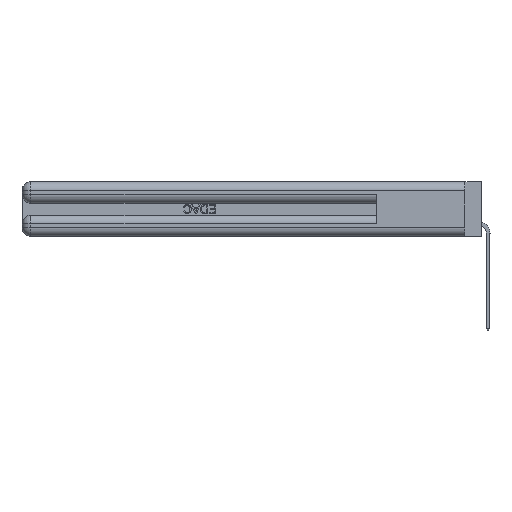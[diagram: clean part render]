
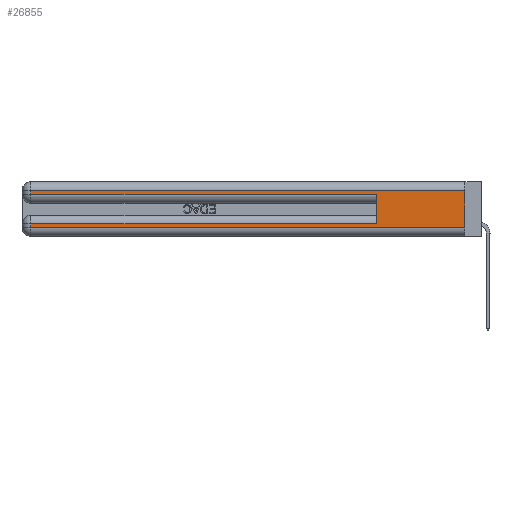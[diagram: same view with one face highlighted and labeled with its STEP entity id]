
A CAD part, left-side view. The second image highlights one B-rep face of the part: STEP entity #26855.
In plain terms, the highlighted planar face has unit normal (-1, 0, 0).
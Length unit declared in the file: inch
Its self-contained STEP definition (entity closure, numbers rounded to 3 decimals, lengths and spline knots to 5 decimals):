
#273 = CARTESIAN_POINT ( 'NONE',  ( 0., 0.6, 0.145 ) ) ;
#765 = ORIENTED_EDGE ( 'NONE', *, *, #25468, .F. ) ;
#1074 = VERTEX_POINT ( 'NONE', #37345 ) ;
#1900 = VECTOR ( 'NONE', #47038, 39.37008 ) ;
#2160 = VECTOR ( 'NONE', #4146, 39.37008 ) ;
#3817 = VECTOR ( 'NONE', #32555, 39.37008 ) ;
#4146 = DIRECTION ( 'NONE',  ( 0., 0., 1. ) ) ;
#4957 = ORIENTED_EDGE ( 'NONE', *, *, #15949, .F. ) ;
#7104 = CARTESIAN_POINT ( 'NONE',  ( 0., 2.94, 0.37 ) ) ;
#8196 = PLANE ( 'NONE',  #9408 ) ;
#8987 = LINE ( 'NONE', #21500, #15284 ) ;
#9408 = AXIS2_PLACEMENT_3D ( 'NONE', #19768, #37480, #22965 ) ;
#9443 = EDGE_LOOP ( 'NONE', ( #765, #43252, #29147, #25705, #4957, #15917, #16515, #45748 ) ) ;
#9847 = VERTEX_POINT ( 'NONE', #37475 ) ;
#10037 = VERTEX_POINT ( 'NONE', #35838 ) ;
#12212 = EDGE_CURVE ( 'NONE', #10037, #40613, #35319, .T. ) ;
#14275 = LINE ( 'NONE', #273, #2160 ) ;
#14607 = LINE ( 'NONE', #45382, #1900 ) ;
#14815 = CARTESIAN_POINT ( 'NONE',  ( 0., 0., 0.285 ) ) ;
#15149 = LINE ( 'NONE', #35776, #22047 ) ;
#15284 = VECTOR ( 'NONE', #17341, 39.37008 ) ;
#15917 = ORIENTED_EDGE ( 'NONE', *, *, #21613, .T. ) ;
#15949 = EDGE_CURVE ( 'NONE', #1074, #41751, #14275, .T. ) ;
#16515 = ORIENTED_EDGE ( 'NONE', *, *, #39843, .T. ) ;
#16596 = VERTEX_POINT ( 'NONE', #25497 ) ;
#17341 = DIRECTION ( 'NONE',  ( 0., 1., 0. ) ) ;
#18153 = VECTOR ( 'NONE', #25629, 39.37008 ) ;
#19569 = VERTEX_POINT ( 'NONE', #19825 ) ;
#19768 = CARTESIAN_POINT ( 'NONE',  ( 0., 0., 0.37 ) ) ;
#19825 = CARTESIAN_POINT ( 'NONE',  ( 0., 2.94, 0.285 ) ) ;
#21500 = CARTESIAN_POINT ( 'NONE',  ( 0., 0., 0.31 ) ) ;
#21613 = EDGE_CURVE ( 'NONE', #1074, #9847, #14607, .T. ) ;
#21876 = DIRECTION ( 'NONE',  ( 0., -1., 0. ) ) ;
#22047 = VECTOR ( 'NONE', #28449, 39.37008 ) ;
#22965 = DIRECTION ( 'NONE',  ( 0., 0., -1. ) ) ;
#23069 = CARTESIAN_POINT ( 'NONE',  ( 0., 0., 0.31 ) ) ;
#23416 = LINE ( 'NONE', #28890, #3817 ) ;
#25326 = EDGE_CURVE ( 'NONE', #19569, #41751, #44003, .T. ) ;
#25468 = EDGE_CURVE ( 'NONE', #39016, #40613, #23416, .T. ) ;
#25497 = CARTESIAN_POINT ( 'NONE',  ( 0., 2.94, 0.31 ) ) ;
#25629 = DIRECTION ( 'NONE',  ( 0., -1., 0. ) ) ;
#25705 = ORIENTED_EDGE ( 'NONE', *, *, #25326, .T. ) ;
#26045 = FACE_OUTER_BOUND ( 'NONE', #9443, .T. ) ;
#26855 = ADVANCED_FACE ( 'NONE', ( #26045 ), #8196, .F. ) ;
#28449 = DIRECTION ( 'NONE',  ( 0., 0., -1. ) ) ;
#28890 = CARTESIAN_POINT ( 'NONE',  ( 0., 0., 0.37 ) ) ;
#29147 = ORIENTED_EDGE ( 'NONE', *, *, #29321, .T. ) ;
#29321 = EDGE_CURVE ( 'NONE', #16596, #19569, #42049, .T. ) ;
#31418 = VECTOR ( 'NONE', #21876, 39.37008 ) ;
#32555 = DIRECTION ( 'NONE',  ( 0., 0., -1. ) ) ;
#34088 = CARTESIAN_POINT ( 'NONE',  ( 0., 0.6, 0.285 ) ) ;
#35319 = LINE ( 'NONE', #42618, #18153 ) ;
#35776 = CARTESIAN_POINT ( 'NONE',  ( 0., 2.94, 0.37 ) ) ;
#35838 = CARTESIAN_POINT ( 'NONE',  ( 0., 2.94, 0.06 ) ) ;
#37345 = CARTESIAN_POINT ( 'NONE',  ( 0., 0.6, 0.085 ) ) ;
#37475 = CARTESIAN_POINT ( 'NONE',  ( 0., 2.94, 0.085 ) ) ;
#37480 = DIRECTION ( 'NONE',  ( 1., 0., 0. ) ) ;
#38726 = EDGE_CURVE ( 'NONE', #39016, #16596, #8987, .T. ) ;
#39016 = VERTEX_POINT ( 'NONE', #23069 ) ;
#39687 = VECTOR ( 'NONE', #47153, 39.37008 ) ;
#39843 = EDGE_CURVE ( 'NONE', #9847, #10037, #15149, .T. ) ;
#40613 = VERTEX_POINT ( 'NONE', #46781 ) ;
#41751 = VERTEX_POINT ( 'NONE', #34088 ) ;
#42049 = LINE ( 'NONE', #7104, #39687 ) ;
#42618 = CARTESIAN_POINT ( 'NONE',  ( 0., 0., 0.06 ) ) ;
#43252 = ORIENTED_EDGE ( 'NONE', *, *, #38726, .T. ) ;
#44003 = LINE ( 'NONE', #14815, #31418 ) ;
#45382 = CARTESIAN_POINT ( 'NONE',  ( 0., 0., 0.085 ) ) ;
#45748 = ORIENTED_EDGE ( 'NONE', *, *, #12212, .T. ) ;
#46781 = CARTESIAN_POINT ( 'NONE',  ( 0., 0., 0.06 ) ) ;
#47038 = DIRECTION ( 'NONE',  ( 0., 1., 0. ) ) ;
#47153 = DIRECTION ( 'NONE',  ( 0., 0., -1. ) ) ;
